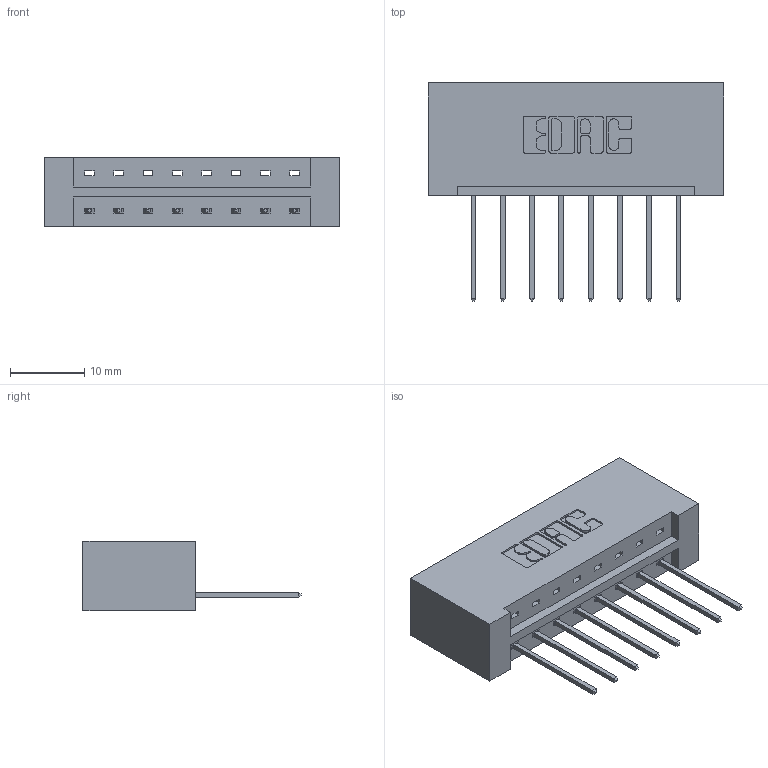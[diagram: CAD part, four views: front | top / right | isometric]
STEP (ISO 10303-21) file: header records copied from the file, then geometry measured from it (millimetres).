
FILE_DESCRIPTION (( 'STEP AP203' ), '1' );
FILE_NAME ('833-008-540-101.STEP', '2020-05-30T16:05:12', ( '' ), ( '' ), 'SwSTEP 2.0', 'SolidWorks 2020', '' );
FILE_SCHEMA (( 'CONFIG_CONTROL_DESIGN' ));
Length unit declared in the file: inch
Products named in the file (3): 345-292-001_345-293-140; 833-008-540-101; 833 Part_Lugless
Assembly tree (9 placements, depth 2):
  833-008-540-101
    833 Part_Lugless
    345-292-001_345-293-140  x8
Bounding box: 39.95 x 29.47 x 9.4 mm (x, y, z)
Volume: 4351.7 mm3; surface area: 4523.3 mm2
Topology: 9 solids, 9 shells, 570 faces, 1695 edges, 1118 vertices
Faces by surface type: plane 402, cylinder 168
Entity records: 9029 total; most frequent: CARTESIAN_POINT 1570, ORIENTED_EDGE 1514, DIRECTION 1385, EDGE_CURVE 757, VECTOR 637, LINE 637, VERTEX_POINT 502, AXIS2_PLACEMENT_3D 374
